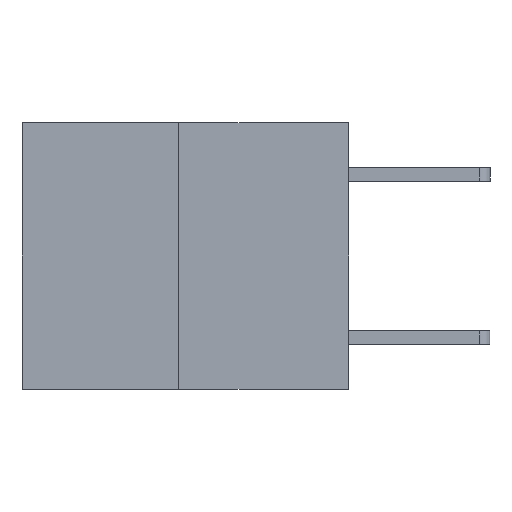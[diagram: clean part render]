
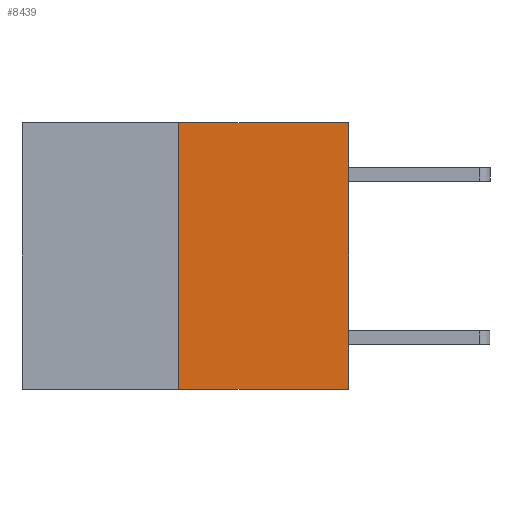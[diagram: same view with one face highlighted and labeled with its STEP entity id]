
A CAD part, left-side view. The second image highlights one B-rep face of the part: STEP entity #8439.
In plain terms, the highlighted planar face has unit normal (-1, 0, 0).
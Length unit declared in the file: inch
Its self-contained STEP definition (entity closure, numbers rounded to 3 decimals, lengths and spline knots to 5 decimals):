
#123 = DIRECTION ( 'NONE',  ( 0., 0., 1. ) ) ;
#445 = ORIENTED_EDGE ( 'NONE', *, *, #4026, .F. ) ;
#497 = CARTESIAN_POINT ( 'NONE',  ( 0., 0., -0.49 ) ) ;
#661 = VECTOR ( 'NONE', #1857, 39.37008 ) ;
#1118 = CARTESIAN_POINT ( 'NONE',  ( 0., 0.6, 0. ) ) ;
#1857 = DIRECTION ( 'NONE',  ( 0., -1., 0. ) ) ;
#1929 = EDGE_CURVE ( 'NONE', #6913, #8664, #2121, .T. ) ;
#2121 = LINE ( 'NONE', #2575, #5113 ) ;
#2223 = EDGE_CURVE ( 'NONE', #6825, #4285, #7656, .T. ) ;
#2494 = EDGE_CURVE ( 'NONE', #6913, #6825, #8958, .T. ) ;
#2499 = CARTESIAN_POINT ( 'NONE',  ( 0., 0.312, 0. ) ) ;
#2575 = CARTESIAN_POINT ( 'NONE',  ( 0., 0.312, -0.49 ) ) ;
#2889 = VECTOR ( 'NONE', #8061, 39.37008 ) ;
#3125 = CARTESIAN_POINT ( 'NONE',  ( 0., 0.6, -0.49 ) ) ;
#3838 = DIRECTION ( 'NONE',  ( 0., 0., 1. ) ) ;
#4026 = EDGE_CURVE ( 'NONE', #8664, #4285, #6319, .T. ) ;
#4285 = VERTEX_POINT ( 'NONE', #4926 ) ;
#4295 = EDGE_LOOP ( 'NONE', ( #7360, #5577, #8780, #445 ) ) ;
#4926 = CARTESIAN_POINT ( 'NONE',  ( 0., 0., 0. ) ) ;
#5113 = VECTOR ( 'NONE', #3838, 39.37008 ) ;
#5577 = ORIENTED_EDGE ( 'NONE', *, *, #2494, .T. ) ;
#5781 = VECTOR ( 'NONE', #123, 39.37008 ) ;
#6319 = LINE ( 'NONE', #1118, #661 ) ;
#6523 = PLANE ( 'NONE',  #8556 ) ;
#6825 = VERTEX_POINT ( 'NONE', #497 ) ;
#6913 = VERTEX_POINT ( 'NONE', #8969 ) ;
#7162 = DIRECTION ( 'NONE',  ( 0., 0., -1. ) ) ;
#7246 = DIRECTION ( 'NONE',  ( 1., 0., 0. ) ) ;
#7360 = ORIENTED_EDGE ( 'NONE', *, *, #1929, .F. ) ;
#7656 = LINE ( 'NONE', #8521, #5781 ) ;
#7875 = CARTESIAN_POINT ( 'NONE',  ( 0., 0.6, 0. ) ) ;
#8061 = DIRECTION ( 'NONE',  ( 0., -1., 0. ) ) ;
#8439 = ADVANCED_FACE ( 'NONE', ( #8854 ), #6523, .F. ) ;
#8521 = CARTESIAN_POINT ( 'NONE',  ( 0., 0., 0. ) ) ;
#8556 = AXIS2_PLACEMENT_3D ( 'NONE', #7875, #7246, #7162 ) ;
#8664 = VERTEX_POINT ( 'NONE', #2499 ) ;
#8780 = ORIENTED_EDGE ( 'NONE', *, *, #2223, .T. ) ;
#8854 = FACE_OUTER_BOUND ( 'NONE', #4295, .T. ) ;
#8958 = LINE ( 'NONE', #3125, #2889 ) ;
#8969 = CARTESIAN_POINT ( 'NONE',  ( 0., 0.312, -0.49 ) ) ;
